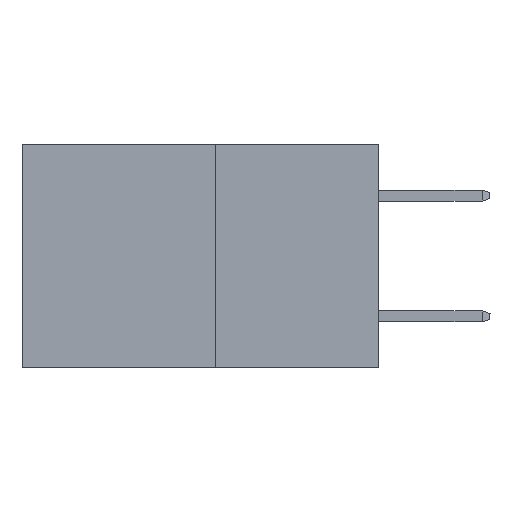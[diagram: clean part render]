
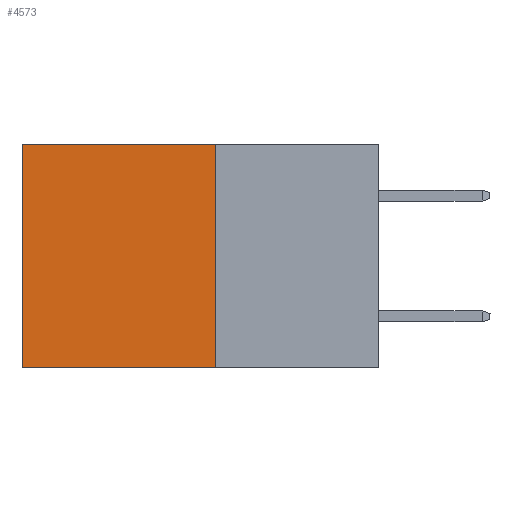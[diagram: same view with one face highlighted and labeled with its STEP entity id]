
A CAD part, left-side view. The second image highlights one B-rep face of the part: STEP entity #4573.
In plain terms, the highlighted planar face has unit normal (-1, 0, 0).
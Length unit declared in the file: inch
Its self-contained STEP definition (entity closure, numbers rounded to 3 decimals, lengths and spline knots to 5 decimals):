
#690 = EDGE_CURVE ( 'NONE', #977, #3266, #7956, .T. ) ;
#789 = DIRECTION ( 'NONE',  ( 0., 1., 0. ) ) ;
#906 = CARTESIAN_POINT ( 'NONE',  ( 0.277, 0.27, 0. ) ) ;
#977 = VERTEX_POINT ( 'NONE', #9136 ) ;
#1019 = VERTEX_POINT ( 'NONE', #906 ) ;
#1474 = CARTESIAN_POINT ( 'NONE',  ( 0.277, 0.59, -0.37 ) ) ;
#1986 = VECTOR ( 'NONE', #12722, 39.37008 ) ;
#2018 = VERTEX_POINT ( 'NONE', #6979 ) ;
#3037 = EDGE_CURVE ( 'NONE', #1019, #2018, #10129, .T. ) ;
#3266 = VERTEX_POINT ( 'NONE', #3537 ) ;
#3296 = DIRECTION ( 'NONE',  ( 0., 0., -1. ) ) ;
#3316 = DIRECTION ( 'NONE',  ( 1., 0., 0. ) ) ;
#3416 = CARTESIAN_POINT ( 'NONE',  ( 0.277, 0.27, -0.37 ) ) ;
#3430 = PLANE ( 'NONE',  #5742 ) ;
#3537 = CARTESIAN_POINT ( 'NONE',  ( 0.277, 0.59, -0.37 ) ) ;
#4573 = ADVANCED_FACE ( 'NONE', ( #11475 ), #3430, .F. ) ;
#5742 = AXIS2_PLACEMENT_3D ( 'NONE', #3416, #3316, #3296 ) ;
#6208 = CARTESIAN_POINT ( 'NONE',  ( 0.277, 0.27, 0. ) ) ;
#6243 = DIRECTION ( 'NONE',  ( 0., 1., 0. ) ) ;
#6482 = EDGE_LOOP ( 'NONE', ( #7262, #12466, #10212, #12745 ) ) ;
#6979 = CARTESIAN_POINT ( 'NONE',  ( 0.277, 0.59, 0. ) ) ;
#7262 = ORIENTED_EDGE ( 'NONE', *, *, #9701, .T. ) ;
#7956 = LINE ( 'NONE', #8218, #8280 ) ;
#7974 = CARTESIAN_POINT ( 'NONE',  ( 0.277, 0.27, -0.37 ) ) ;
#8218 = CARTESIAN_POINT ( 'NONE',  ( 0.277, 0.27, -0.37 ) ) ;
#8280 = VECTOR ( 'NONE', #789, 39.37008 ) ;
#8530 = LINE ( 'NONE', #7974, #10524 ) ;
#8970 = DIRECTION ( 'NONE',  ( 0., 0., -1. ) ) ;
#9136 = CARTESIAN_POINT ( 'NONE',  ( 0.277, 0.27, -0.37 ) ) ;
#9230 = VECTOR ( 'NONE', #6243, 39.37008 ) ;
#9701 = EDGE_CURVE ( 'NONE', #2018, #3266, #10607, .T. ) ;
#10129 = LINE ( 'NONE', #6208, #9230 ) ;
#10212 = ORIENTED_EDGE ( 'NONE', *, *, #12652, .F. ) ;
#10524 = VECTOR ( 'NONE', #8970, 39.37008 ) ;
#10607 = LINE ( 'NONE', #1474, #1986 ) ;
#11475 = FACE_OUTER_BOUND ( 'NONE', #6482, .T. ) ;
#12466 = ORIENTED_EDGE ( 'NONE', *, *, #690, .F. ) ;
#12652 = EDGE_CURVE ( 'NONE', #1019, #977, #8530, .T. ) ;
#12722 = DIRECTION ( 'NONE',  ( 0., 0., -1. ) ) ;
#12745 = ORIENTED_EDGE ( 'NONE', *, *, #3037, .T. ) ;
